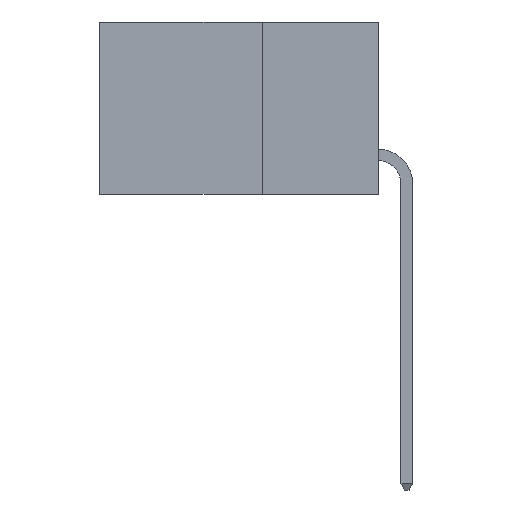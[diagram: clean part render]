
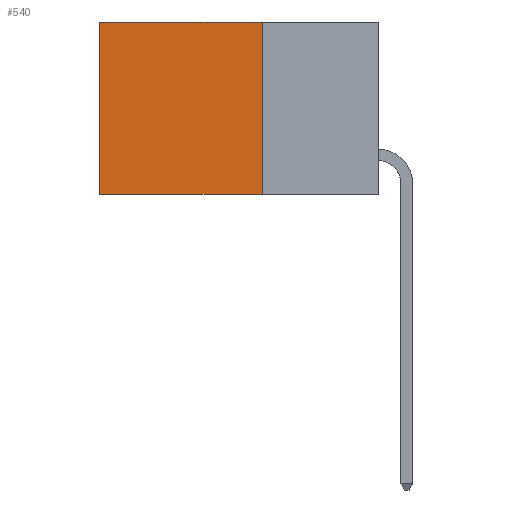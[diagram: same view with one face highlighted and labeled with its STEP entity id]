
A CAD part, left-side view. The second image highlights one B-rep face of the part: STEP entity #540.
In plain terms, the highlighted planar face has unit normal (-1, 0, 0).
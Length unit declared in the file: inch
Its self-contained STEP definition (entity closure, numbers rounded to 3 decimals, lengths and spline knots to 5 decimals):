
#435 = VERTEX_POINT ( 'NONE', #20100 ) ;
#540 = ADVANCED_FACE ( 'NONE', ( #7673 ), #17651, .F. ) ;
#935 = EDGE_CURVE ( 'NONE', #435, #3615, #12472, .T. ) ;
#1575 = VECTOR ( 'NONE', #9278, 39.37008 ) ;
#1627 = LINE ( 'NONE', #7614, #10548 ) ;
#3615 = VERTEX_POINT ( 'NONE', #10589 ) ;
#6439 = EDGE_CURVE ( 'NONE', #435, #21801, #20526, .T. ) ;
#7374 = ORIENTED_EDGE ( 'NONE', *, *, #11872, .F. ) ;
#7542 = DIRECTION ( 'NONE',  ( 0., 1., 0. ) ) ;
#7556 = DIRECTION ( 'NONE',  ( 0., 0., -1. ) ) ;
#7614 = CARTESIAN_POINT ( 'NONE',  ( 0.2615, 0.25, -0.37 ) ) ;
#7663 = DIRECTION ( 'NONE',  ( 0., 0., -1. ) ) ;
#7673 = FACE_OUTER_BOUND ( 'NONE', #14488, .T. ) ;
#7685 = CARTESIAN_POINT ( 'NONE',  ( 0.2615, 0.6, -0.37 ) ) ;
#7755 = DIRECTION ( 'NONE',  ( 0., 0., -1. ) ) ;
#9278 = DIRECTION ( 'NONE',  ( 0., 1., 0. ) ) ;
#10081 = AXIS2_PLACEMENT_3D ( 'NONE', #15294, #15227, #7556 ) ;
#10548 = VECTOR ( 'NONE', #7542, 39.37008 ) ;
#10589 = CARTESIAN_POINT ( 'NONE',  ( 0.2615, 0.25, -0.37 ) ) ;
#10603 = VERTEX_POINT ( 'NONE', #20895 ) ;
#11617 = CARTESIAN_POINT ( 'NONE',  ( 0.2615, 0.25, 0. ) ) ;
#11833 = EDGE_CURVE ( 'NONE', #21801, #10603, #15954, .T. ) ;
#11872 = EDGE_CURVE ( 'NONE', #3615, #10603, #1627, .T. ) ;
#12472 = LINE ( 'NONE', #16760, #21282 ) ;
#14488 = EDGE_LOOP ( 'NONE', ( #15941, #7374, #14747, #20155 ) ) ;
#14747 = ORIENTED_EDGE ( 'NONE', *, *, #935, .F. ) ;
#15227 = DIRECTION ( 'NONE',  ( 1., 0., 0. ) ) ;
#15294 = CARTESIAN_POINT ( 'NONE',  ( 0.2615, 0.25, -0.37 ) ) ;
#15941 = ORIENTED_EDGE ( 'NONE', *, *, #11833, .T. ) ;
#15954 = LINE ( 'NONE', #7685, #20577 ) ;
#16760 = CARTESIAN_POINT ( 'NONE',  ( 0.2615, 0.25, -0.37 ) ) ;
#17178 = CARTESIAN_POINT ( 'NONE',  ( 0.2615, 0.6, 0. ) ) ;
#17651 = PLANE ( 'NONE',  #10081 ) ;
#20100 = CARTESIAN_POINT ( 'NONE',  ( 0.2615, 0.25, 0. ) ) ;
#20155 = ORIENTED_EDGE ( 'NONE', *, *, #6439, .T. ) ;
#20526 = LINE ( 'NONE', #11617, #1575 ) ;
#20577 = VECTOR ( 'NONE', #7663, 39.37008 ) ;
#20895 = CARTESIAN_POINT ( 'NONE',  ( 0.2615, 0.6, -0.37 ) ) ;
#21282 = VECTOR ( 'NONE', #7755, 39.37008 ) ;
#21801 = VERTEX_POINT ( 'NONE', #17178 ) ;
